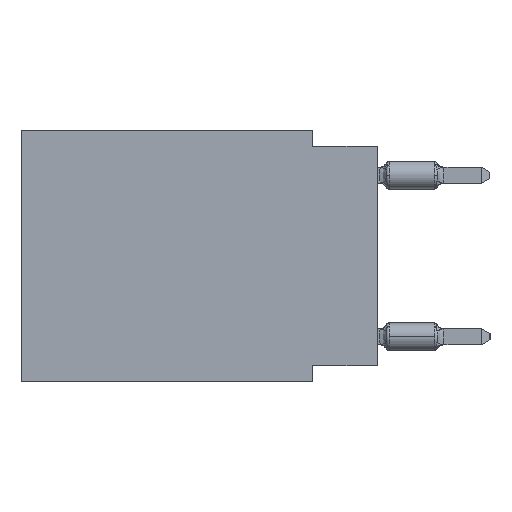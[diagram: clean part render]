
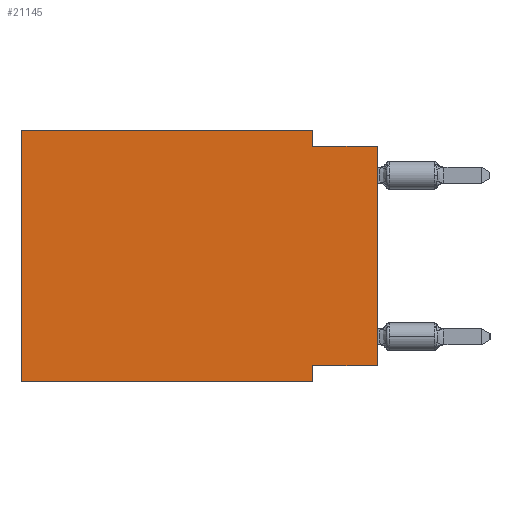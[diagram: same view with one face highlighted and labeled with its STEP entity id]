
A CAD part, left-side view. The second image highlights one B-rep face of the part: STEP entity #21145.
In plain terms, the highlighted planar face has unit normal (-1, 0, 0).
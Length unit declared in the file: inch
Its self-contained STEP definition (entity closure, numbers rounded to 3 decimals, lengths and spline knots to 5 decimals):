
#469 = VERTEX_POINT ( 'NONE', #2453 ) ;
#592 = VERTEX_POINT ( 'NONE', #9295 ) ;
#680 = CARTESIAN_POINT ( 'NONE',  ( 0., 0.55, -0.39 ) ) ;
#717 = LINE ( 'NONE', #6294, #8374 ) ;
#1489 = LINE ( 'NONE', #17286, #21047 ) ;
#2330 = VERTEX_POINT ( 'NONE', #15985 ) ;
#2453 = CARTESIAN_POINT ( 'NONE',  ( 0., 0.1, -0.365 ) ) ;
#2728 = VECTOR ( 'NONE', #14081, 39.37008 ) ;
#3742 = EDGE_CURVE ( 'NONE', #592, #12850, #9658, .T. ) ;
#3776 = AXIS2_PLACEMENT_3D ( 'NONE', #22182, #23735, #4054 ) ;
#3805 = LINE ( 'NONE', #10023, #21471 ) ;
#4018 = ORIENTED_EDGE ( 'NONE', *, *, #6530, .T. ) ;
#4054 = DIRECTION ( 'NONE',  ( 0., 0., -1. ) ) ;
#5006 = VECTOR ( 'NONE', #5286, 39.37008 ) ;
#5286 = DIRECTION ( 'NONE',  ( 0., 0., 1. ) ) ;
#5434 = CARTESIAN_POINT ( 'NONE',  ( 0., 0.1, -0.025 ) ) ;
#5492 = VERTEX_POINT ( 'NONE', #5434 ) ;
#6294 = CARTESIAN_POINT ( 'NONE',  ( 0., 0.1, -0.39 ) ) ;
#6530 = EDGE_CURVE ( 'NONE', #22136, #6825, #18416, .T. ) ;
#6825 = VERTEX_POINT ( 'NONE', #18121 ) ;
#7118 = VECTOR ( 'NONE', #16841, 39.37008 ) ;
#7229 = LINE ( 'NONE', #15103, #5006 ) ;
#7601 = DIRECTION ( 'NONE',  ( 0., 1., 0. ) ) ;
#7888 = CARTESIAN_POINT ( 'NONE',  ( 0., 0.55, 0. ) ) ;
#8146 = LINE ( 'NONE', #24197, #2728 ) ;
#8374 = VECTOR ( 'NONE', #24544, 39.37008 ) ;
#8914 = ORIENTED_EDGE ( 'NONE', *, *, #15468, .F. ) ;
#9295 = CARTESIAN_POINT ( 'NONE',  ( 0., 0.55, 0. ) ) ;
#9658 = LINE ( 'NONE', #17535, #11103 ) ;
#10023 = CARTESIAN_POINT ( 'NONE',  ( 0., 0., -0.025 ) ) ;
#10126 = ORIENTED_EDGE ( 'NONE', *, *, #20586, .T. ) ;
#10218 = ORIENTED_EDGE ( 'NONE', *, *, #17651, .F. ) ;
#11103 = VECTOR ( 'NONE', #25419, 39.37008 ) ;
#11955 = DIRECTION ( 'NONE',  ( 0., -1., 0. ) ) ;
#12059 = ORIENTED_EDGE ( 'NONE', *, *, #3742, .F. ) ;
#12159 = LINE ( 'NONE', #7888, #23479 ) ;
#12608 = ORIENTED_EDGE ( 'NONE', *, *, #17063, .F. ) ;
#12728 = EDGE_CURVE ( 'NONE', #12850, #5492, #8146, .T. ) ;
#12850 = VERTEX_POINT ( 'NONE', #16288 ) ;
#13411 = CARTESIAN_POINT ( 'NONE',  ( 0., 0.55, -0.39 ) ) ;
#14081 = DIRECTION ( 'NONE',  ( 0., 0., -1. ) ) ;
#15103 = CARTESIAN_POINT ( 'NONE',  ( 0., 0., 0. ) ) ;
#15468 = EDGE_CURVE ( 'NONE', #22136, #592, #12159, .T. ) ;
#15763 = DIRECTION ( 'NONE',  ( 0., 0., 1. ) ) ;
#15949 = PLANE ( 'NONE',  #3776 ) ;
#15952 = VERTEX_POINT ( 'NONE', #21423 ) ;
#15985 = CARTESIAN_POINT ( 'NONE',  ( 0., 0., -0.025 ) ) ;
#16288 = CARTESIAN_POINT ( 'NONE',  ( 0., 0.1, 0. ) ) ;
#16841 = DIRECTION ( 'NONE',  ( 0., -1., 0. ) ) ;
#17063 = EDGE_CURVE ( 'NONE', #15952, #469, #1489, .T. ) ;
#17286 = CARTESIAN_POINT ( 'NONE',  ( 0., 0., -0.365 ) ) ;
#17535 = CARTESIAN_POINT ( 'NONE',  ( 0., 0.55, 0. ) ) ;
#17651 = EDGE_CURVE ( 'NONE', #5492, #2330, #3805, .T. ) ;
#18121 = CARTESIAN_POINT ( 'NONE',  ( 0., 0.1, -0.39 ) ) ;
#18286 = FACE_OUTER_BOUND ( 'NONE', #19470, .T. ) ;
#18416 = LINE ( 'NONE', #680, #7118 ) ;
#19470 = EDGE_LOOP ( 'NONE', ( #10126, #10218, #19593, #12059, #8914, #4018, #23065, #12608 ) ) ;
#19593 = ORIENTED_EDGE ( 'NONE', *, *, #12728, .F. ) ;
#20586 = EDGE_CURVE ( 'NONE', #15952, #2330, #7229, .T. ) ;
#21047 = VECTOR ( 'NONE', #7601, 39.37008 ) ;
#21145 = ADVANCED_FACE ( 'NONE', ( #18286 ), #15949, .F. ) ;
#21423 = CARTESIAN_POINT ( 'NONE',  ( 0., 0., -0.365 ) ) ;
#21471 = VECTOR ( 'NONE', #11955, 39.37008 ) ;
#22136 = VERTEX_POINT ( 'NONE', #13411 ) ;
#22182 = CARTESIAN_POINT ( 'NONE',  ( 0., 0.55, 0. ) ) ;
#22466 = EDGE_CURVE ( 'NONE', #469, #6825, #717, .T. ) ;
#23065 = ORIENTED_EDGE ( 'NONE', *, *, #22466, .F. ) ;
#23479 = VECTOR ( 'NONE', #15763, 39.37008 ) ;
#23735 = DIRECTION ( 'NONE',  ( 1., 0., 0. ) ) ;
#24197 = CARTESIAN_POINT ( 'NONE',  ( 0., 0.1, 0. ) ) ;
#24544 = DIRECTION ( 'NONE',  ( 0., 0., -1. ) ) ;
#25419 = DIRECTION ( 'NONE',  ( 0., -1., 0. ) ) ;
